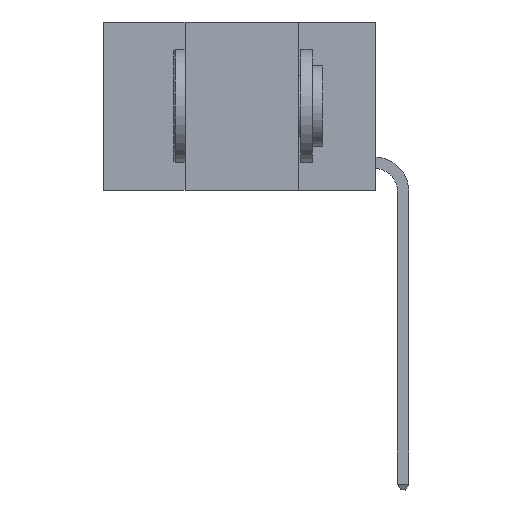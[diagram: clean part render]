
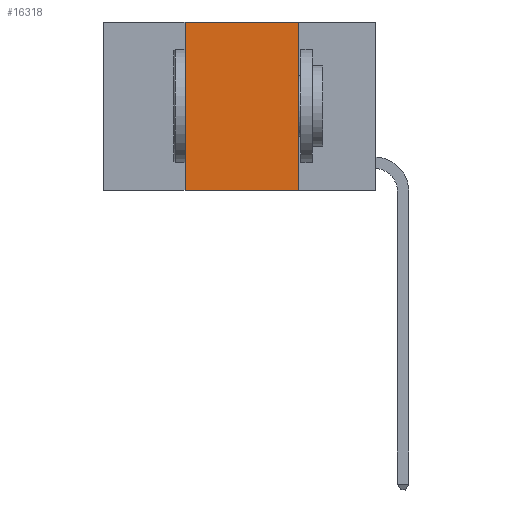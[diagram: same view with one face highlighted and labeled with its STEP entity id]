
A CAD part, left-side view. The second image highlights one B-rep face of the part: STEP entity #16318.
In plain terms, the highlighted planar face has unit normal (-1, 0, 0).
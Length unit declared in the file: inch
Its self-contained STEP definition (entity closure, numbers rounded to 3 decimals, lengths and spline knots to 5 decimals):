
#425 = CARTESIAN_POINT ( 'NONE',  ( 0., 0.42, 0. ) ) ;
#650 = ORIENTED_EDGE ( 'NONE', *, *, #16709, .F. ) ;
#860 = EDGE_CURVE ( 'NONE', #8563, #20117, #9057, .T. ) ;
#1702 = DIRECTION ( 'NONE',  ( 0., -1., 0. ) ) ;
#2749 = EDGE_CURVE ( 'NONE', #13463, #19487, #8813, .T. ) ;
#4008 = CARTESIAN_POINT ( 'NONE',  ( 0., 0.6, -0.37 ) ) ;
#4848 = ORIENTED_EDGE ( 'NONE', *, *, #860, .F. ) ;
#5456 = DIRECTION ( 'NONE',  ( 0., 0., 1. ) ) ;
#5607 = VECTOR ( 'NONE', #20934, 39.37008 ) ;
#7179 = VECTOR ( 'NONE', #1702, 39.37008 ) ;
#8563 = VERTEX_POINT ( 'NONE', #11055 ) ;
#8813 = LINE ( 'NONE', #16875, #17259 ) ;
#9057 = LINE ( 'NONE', #12615, #5607 ) ;
#11055 = CARTESIAN_POINT ( 'NONE',  ( 0., 0.17, 0. ) ) ;
#11621 = VECTOR ( 'NONE', #19983, 39.37008 ) ;
#12378 = LINE ( 'NONE', #4008, #11621 ) ;
#12615 = CARTESIAN_POINT ( 'NONE',  ( 0., 0.17, 0. ) ) ;
#13150 = ORIENTED_EDGE ( 'NONE', *, *, #16059, .T. ) ;
#13200 = EDGE_LOOP ( 'NONE', ( #4848, #650, #20973, #13150 ) ) ;
#13463 = VERTEX_POINT ( 'NONE', #15246 ) ;
#14772 = DIRECTION ( 'NONE',  ( 1., 0., 0. ) ) ;
#14892 = FACE_OUTER_BOUND ( 'NONE', #13200, .T. ) ;
#14997 = CARTESIAN_POINT ( 'NONE',  ( 0., 0.6, 0. ) ) ;
#15246 = CARTESIAN_POINT ( 'NONE',  ( 0., 0.42, -0.37 ) ) ;
#16015 = CARTESIAN_POINT ( 'NONE',  ( 0., 0.17, -0.37 ) ) ;
#16059 = EDGE_CURVE ( 'NONE', #13463, #20117, #12378, .T. ) ;
#16318 = ADVANCED_FACE ( 'NONE', ( #14892 ), #21336, .F. ) ;
#16406 = DIRECTION ( 'NONE',  ( 0., 0., -1. ) ) ;
#16709 = EDGE_CURVE ( 'NONE', #19487, #8563, #19462, .T. ) ;
#16875 = CARTESIAN_POINT ( 'NONE',  ( 0., 0.42, 0. ) ) ;
#17259 = VECTOR ( 'NONE', #5456, 39.37008 ) ;
#18654 = AXIS2_PLACEMENT_3D ( 'NONE', #14997, #14772, #16406 ) ;
#19462 = LINE ( 'NONE', #21302, #7179 ) ;
#19487 = VERTEX_POINT ( 'NONE', #425 ) ;
#19983 = DIRECTION ( 'NONE',  ( 0., -1., 0. ) ) ;
#20117 = VERTEX_POINT ( 'NONE', #16015 ) ;
#20934 = DIRECTION ( 'NONE',  ( 0., 0., -1. ) ) ;
#20973 = ORIENTED_EDGE ( 'NONE', *, *, #2749, .F. ) ;
#21302 = CARTESIAN_POINT ( 'NONE',  ( 0., 0.6, 0. ) ) ;
#21336 = PLANE ( 'NONE',  #18654 ) ;
